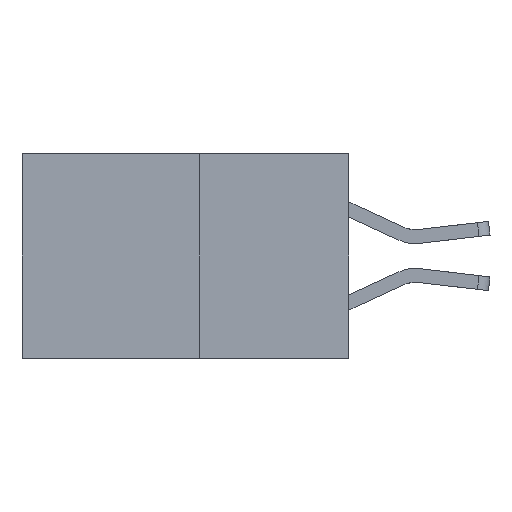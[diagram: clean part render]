
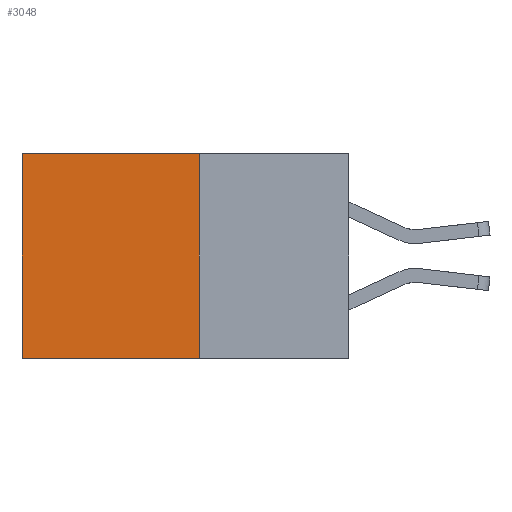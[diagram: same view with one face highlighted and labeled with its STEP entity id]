
A CAD part, left-side view. The second image highlights one B-rep face of the part: STEP entity #3048.
In plain terms, the highlighted planar face has unit normal (-1, 0, 0).
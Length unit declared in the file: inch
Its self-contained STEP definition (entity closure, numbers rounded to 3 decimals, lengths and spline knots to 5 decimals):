
#37 = CARTESIAN_POINT ( 'NONE',  ( 0.277, 0.27, 0. ) ) ;
#517 = AXIS2_PLACEMENT_3D ( 'NONE', #5387, #3774, #2337 ) ;
#750 = CARTESIAN_POINT ( 'NONE',  ( 0.277, 0.27, -0.37 ) ) ;
#830 = ORIENTED_EDGE ( 'NONE', *, *, #7755, .F. ) ;
#906 = DIRECTION ( 'NONE',  ( 0., 1., 0. ) ) ;
#999 = DIRECTION ( 'NONE',  ( 0., 0., -1. ) ) ;
#1031 = CARTESIAN_POINT ( 'NONE',  ( 0.277, 0.59, -0.37 ) ) ;
#1202 = CARTESIAN_POINT ( 'NONE',  ( 0.277, 0.27, -0.37 ) ) ;
#1379 = ORIENTED_EDGE ( 'NONE', *, *, #8082, .F. ) ;
#1545 = LINE ( 'NONE', #750, #7292 ) ;
#1995 = CARTESIAN_POINT ( 'NONE',  ( 0.277, 0.59, 0. ) ) ;
#2337 = DIRECTION ( 'NONE',  ( 0., 0., -1. ) ) ;
#2806 = VECTOR ( 'NONE', #4234, 39.37008 ) ;
#3048 = ADVANCED_FACE ( 'NONE', ( #5461 ), #4402, .F. ) ;
#3101 = CARTESIAN_POINT ( 'NONE',  ( 0.277, 0.59, -0.37 ) ) ;
#3429 = LINE ( 'NONE', #7803, #7284 ) ;
#3774 = DIRECTION ( 'NONE',  ( 1., 0., 0. ) ) ;
#3847 = CARTESIAN_POINT ( 'NONE',  ( 0.277, 0.27, -0.37 ) ) ;
#4234 = DIRECTION ( 'NONE',  ( 0., 0., -1. ) ) ;
#4402 = PLANE ( 'NONE',  #517 ) ;
#4548 = VERTEX_POINT ( 'NONE', #3101 ) ;
#5366 = VERTEX_POINT ( 'NONE', #1995 ) ;
#5387 = CARTESIAN_POINT ( 'NONE',  ( 0.277, 0.27, -0.37 ) ) ;
#5461 = FACE_OUTER_BOUND ( 'NONE', #9708, .T. ) ;
#6733 = VECTOR ( 'NONE', #999, 39.37008 ) ;
#7284 = VECTOR ( 'NONE', #7945, 39.37008 ) ;
#7292 = VECTOR ( 'NONE', #906, 39.37008 ) ;
#7709 = EDGE_CURVE ( 'NONE', #5366, #4548, #9591, .T. ) ;
#7755 = EDGE_CURVE ( 'NONE', #8046, #4548, #1545, .T. ) ;
#7803 = CARTESIAN_POINT ( 'NONE',  ( 0.277, 0.27, 0. ) ) ;
#7932 = VERTEX_POINT ( 'NONE', #37 ) ;
#7945 = DIRECTION ( 'NONE',  ( 0., 1., 0. ) ) ;
#8046 = VERTEX_POINT ( 'NONE', #3847 ) ;
#8082 = EDGE_CURVE ( 'NONE', #7932, #8046, #8660, .T. ) ;
#8266 = EDGE_CURVE ( 'NONE', #7932, #5366, #3429, .T. ) ;
#8596 = ORIENTED_EDGE ( 'NONE', *, *, #7709, .T. ) ;
#8660 = LINE ( 'NONE', #1202, #2806 ) ;
#8710 = ORIENTED_EDGE ( 'NONE', *, *, #8266, .T. ) ;
#9591 = LINE ( 'NONE', #1031, #6733 ) ;
#9708 = EDGE_LOOP ( 'NONE', ( #8596, #830, #1379, #8710 ) ) ;
